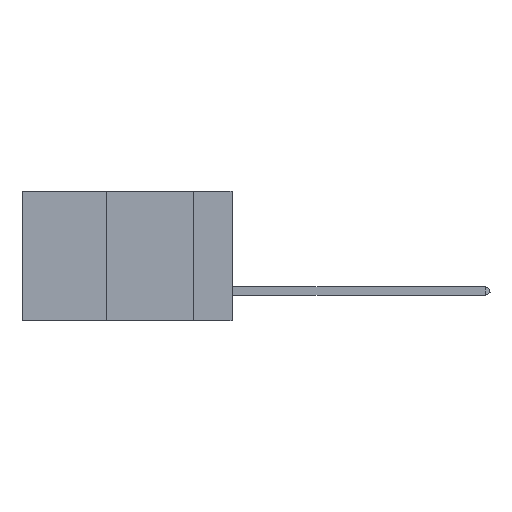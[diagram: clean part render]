
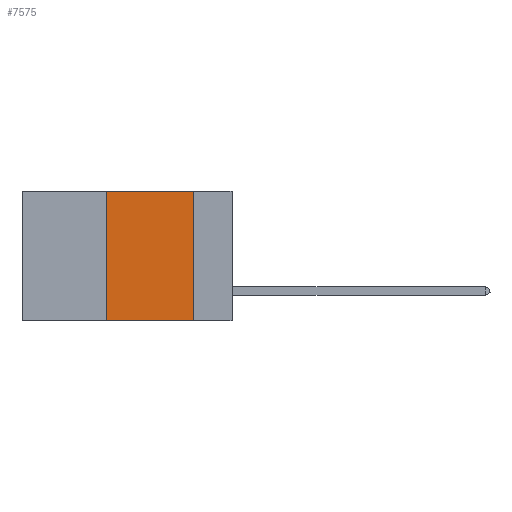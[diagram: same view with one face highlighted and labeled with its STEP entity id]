
A CAD part, left-side view. The second image highlights one B-rep face of the part: STEP entity #7575.
In plain terms, the highlighted planar face has unit normal (-1, 0, 0).
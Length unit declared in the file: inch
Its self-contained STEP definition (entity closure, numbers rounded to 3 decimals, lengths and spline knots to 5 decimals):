
#3192 = CARTESIAN_POINT ( 'NONE',  ( 0., 0.6, -0.37 ) ) ;
#6992 = EDGE_CURVE ( 'NONE', #14526, #24137, #8249, .T. ) ;
#7575 = ADVANCED_FACE ( 'NONE', ( #35356 ), #44937, .F. ) ;
#8249 = LINE ( 'NONE', #12541, #20027 ) ;
#11411 = LINE ( 'NONE', #3192, #47613 ) ;
#12232 = CARTESIAN_POINT ( 'NONE',  ( 0., 0.11, 0. ) ) ;
#12500 = CARTESIAN_POINT ( 'NONE',  ( 0., 0.6, 0. ) ) ;
#12541 = CARTESIAN_POINT ( 'NONE',  ( 0., 0.6, 0. ) ) ;
#13776 = ORIENTED_EDGE ( 'NONE', *, *, #6992, .F. ) ;
#14526 = VERTEX_POINT ( 'NONE', #33041 ) ;
#16258 = DIRECTION ( 'NONE',  ( 0., 0., -1. ) ) ;
#18649 = CARTESIAN_POINT ( 'NONE',  ( 0., 0.36, -0.37 ) ) ;
#19751 = DIRECTION ( 'NONE',  ( 0., -1., 0. ) ) ;
#20027 = VECTOR ( 'NONE', #19751, 39.37008 ) ;
#20692 = ORIENTED_EDGE ( 'NONE', *, *, #42668, .T. ) ;
#21215 = CARTESIAN_POINT ( 'NONE',  ( 0., 0.11, -0.37 ) ) ;
#21523 = VERTEX_POINT ( 'NONE', #21215 ) ;
#21926 = EDGE_LOOP ( 'NONE', ( #34662, #13776, #31608, #20692 ) ) ;
#22074 = DIRECTION ( 'NONE',  ( 0., 0., -1. ) ) ;
#22489 = CARTESIAN_POINT ( 'NONE',  ( 0., 0.36, 0. ) ) ;
#23360 = DIRECTION ( 'NONE',  ( 0., -1., 0. ) ) ;
#24137 = VERTEX_POINT ( 'NONE', #12232 ) ;
#26670 = VECTOR ( 'NONE', #22074, 39.37008 ) ;
#27499 = EDGE_CURVE ( 'NONE', #24137, #21523, #34847, .T. ) ;
#27815 = VECTOR ( 'NONE', #30487, 39.37008 ) ;
#27883 = AXIS2_PLACEMENT_3D ( 'NONE', #12500, #38620, #16258 ) ;
#28338 = LINE ( 'NONE', #22489, #27815 ) ;
#30487 = DIRECTION ( 'NONE',  ( 0., 0., 1. ) ) ;
#31608 = ORIENTED_EDGE ( 'NONE', *, *, #38826, .F. ) ;
#33041 = CARTESIAN_POINT ( 'NONE',  ( 0., 0.36, 0. ) ) ;
#34662 = ORIENTED_EDGE ( 'NONE', *, *, #27499, .F. ) ;
#34847 = LINE ( 'NONE', #46950, #26670 ) ;
#35356 = FACE_OUTER_BOUND ( 'NONE', #21926, .T. ) ;
#38620 = DIRECTION ( 'NONE',  ( 1., 0., 0. ) ) ;
#38826 = EDGE_CURVE ( 'NONE', #46596, #14526, #28338, .T. ) ;
#42668 = EDGE_CURVE ( 'NONE', #46596, #21523, #11411, .T. ) ;
#44937 = PLANE ( 'NONE',  #27883 ) ;
#46596 = VERTEX_POINT ( 'NONE', #18649 ) ;
#46950 = CARTESIAN_POINT ( 'NONE',  ( 0., 0.11, 0. ) ) ;
#47613 = VECTOR ( 'NONE', #23360, 39.37008 ) ;
